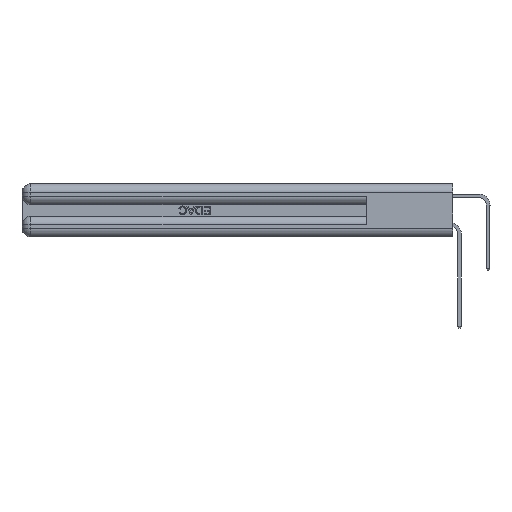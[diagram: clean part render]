
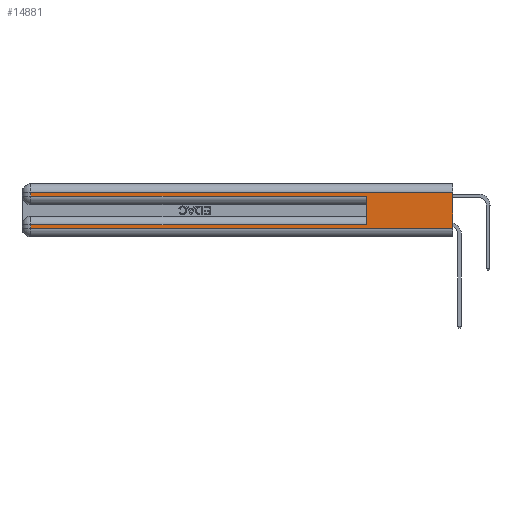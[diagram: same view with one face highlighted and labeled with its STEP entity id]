
A CAD part, left-side view. The second image highlights one B-rep face of the part: STEP entity #14881.
In plain terms, the highlighted planar face has unit normal (-1, 0, 0).
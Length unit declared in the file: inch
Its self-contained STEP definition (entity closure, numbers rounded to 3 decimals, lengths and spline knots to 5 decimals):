
#551 = LINE ( 'NONE', #1925, #33807 ) ;
#1925 = CARTESIAN_POINT ( 'NONE',  ( 0., 0., 0.085 ) ) ;
#4044 = DIRECTION ( 'NONE',  ( 1., 0., 0. ) ) ;
#4581 = CARTESIAN_POINT ( 'NONE',  ( 0., 2.94, 0.31 ) ) ;
#5398 = VERTEX_POINT ( 'NONE', #27032 ) ;
#6913 = LINE ( 'NONE', #38090, #45396 ) ;
#7107 = VERTEX_POINT ( 'NONE', #21104 ) ;
#8309 = CARTESIAN_POINT ( 'NONE',  ( 0., 0., 0.31 ) ) ;
#8334 = ORIENTED_EDGE ( 'NONE', *, *, #34138, .T. ) ;
#8689 = VERTEX_POINT ( 'NONE', #4581 ) ;
#9013 = CARTESIAN_POINT ( 'NONE',  ( 0., 2.94, 0.06 ) ) ;
#9107 = LINE ( 'NONE', #22734, #41726 ) ;
#9156 = VECTOR ( 'NONE', #30788, 39.37008 ) ;
#10543 = EDGE_CURVE ( 'NONE', #7107, #8689, #37160, .T. ) ;
#13018 = DIRECTION ( 'NONE',  ( 0., 1., 0. ) ) ;
#14821 = CARTESIAN_POINT ( 'NONE',  ( 0., 0., 0.37 ) ) ;
#14881 = ADVANCED_FACE ( 'NONE', ( #30387 ), #41164, .F. ) ;
#16146 = DIRECTION ( 'NONE',  ( 0., 0., -1. ) ) ;
#16802 = VERTEX_POINT ( 'NONE', #31632 ) ;
#17012 = VECTOR ( 'NONE', #28247, 39.37008 ) ;
#17228 = ORIENTED_EDGE ( 'NONE', *, *, #10543, .T. ) ;
#17776 = LINE ( 'NONE', #38113, #46366 ) ;
#18522 = VERTEX_POINT ( 'NONE', #23057 ) ;
#19161 = ORIENTED_EDGE ( 'NONE', *, *, #26163, .F. ) ;
#21009 = EDGE_LOOP ( 'NONE', ( #34911, #17228, #40015, #8334, #19161, #46588, #28971, #39958 ) ) ;
#21104 = CARTESIAN_POINT ( 'NONE',  ( 0., 0., 0.31 ) ) ;
#21581 = LINE ( 'NONE', #47509, #40248 ) ;
#22438 = DIRECTION ( 'NONE',  ( 0., 0., -1. ) ) ;
#22734 = CARTESIAN_POINT ( 'NONE',  ( 0., 0., 0.06 ) ) ;
#23057 = CARTESIAN_POINT ( 'NONE',  ( 0., 0.6, 0.085 ) ) ;
#24514 = VERTEX_POINT ( 'NONE', #9013 ) ;
#24845 = AXIS2_PLACEMENT_3D ( 'NONE', #14821, #4044, #22438 ) ;
#25938 = LINE ( 'NONE', #42338, #39953 ) ;
#26163 = EDGE_CURVE ( 'NONE', #18522, #28656, #21581, .T. ) ;
#27032 = CARTESIAN_POINT ( 'NONE',  ( 0., 0., 0.06 ) ) ;
#27153 = EDGE_CURVE ( 'NONE', #7107, #5398, #6913, .T. ) ;
#28247 = DIRECTION ( 'NONE',  ( 0., -1., 0. ) ) ;
#28656 = VERTEX_POINT ( 'NONE', #34473 ) ;
#28904 = DIRECTION ( 'NONE',  ( 0., 0., 1. ) ) ;
#28971 = ORIENTED_EDGE ( 'NONE', *, *, #31458, .T. ) ;
#29905 = DIRECTION ( 'NONE',  ( 0., -1., 0. ) ) ;
#30387 = FACE_OUTER_BOUND ( 'NONE', #21009, .T. ) ;
#30755 = DIRECTION ( 'NONE',  ( 0., 0., -1. ) ) ;
#30788 = DIRECTION ( 'NONE',  ( 0., 1., 0. ) ) ;
#31458 = EDGE_CURVE ( 'NONE', #16802, #24514, #17776, .T. ) ;
#31632 = CARTESIAN_POINT ( 'NONE',  ( 0., 2.94, 0.085 ) ) ;
#33807 = VECTOR ( 'NONE', #13018, 39.37008 ) ;
#34138 = EDGE_CURVE ( 'NONE', #34384, #28656, #35057, .T. ) ;
#34384 = VERTEX_POINT ( 'NONE', #48258 ) ;
#34473 = CARTESIAN_POINT ( 'NONE',  ( 0., 0.6, 0.285 ) ) ;
#34911 = ORIENTED_EDGE ( 'NONE', *, *, #27153, .F. ) ;
#35057 = LINE ( 'NONE', #38888, #17012 ) ;
#37160 = LINE ( 'NONE', #8309, #9156 ) ;
#37734 = EDGE_CURVE ( 'NONE', #18522, #16802, #551, .T. ) ;
#38090 = CARTESIAN_POINT ( 'NONE',  ( 0., 0., 0.37 ) ) ;
#38113 = CARTESIAN_POINT ( 'NONE',  ( 0., 2.94, 0.37 ) ) ;
#38888 = CARTESIAN_POINT ( 'NONE',  ( 0., 0., 0.285 ) ) ;
#39953 = VECTOR ( 'NONE', #46259, 39.37008 ) ;
#39958 = ORIENTED_EDGE ( 'NONE', *, *, #40768, .T. ) ;
#40015 = ORIENTED_EDGE ( 'NONE', *, *, #45877, .T. ) ;
#40248 = VECTOR ( 'NONE', #28904, 39.37008 ) ;
#40768 = EDGE_CURVE ( 'NONE', #24514, #5398, #9107, .T. ) ;
#41164 = PLANE ( 'NONE',  #24845 ) ;
#41726 = VECTOR ( 'NONE', #29905, 39.37008 ) ;
#42338 = CARTESIAN_POINT ( 'NONE',  ( 0., 2.94, 0.37 ) ) ;
#45396 = VECTOR ( 'NONE', #30755, 39.37008 ) ;
#45877 = EDGE_CURVE ( 'NONE', #8689, #34384, #25938, .T. ) ;
#46259 = DIRECTION ( 'NONE',  ( 0., 0., -1. ) ) ;
#46366 = VECTOR ( 'NONE', #16146, 39.37008 ) ;
#46588 = ORIENTED_EDGE ( 'NONE', *, *, #37734, .T. ) ;
#47509 = CARTESIAN_POINT ( 'NONE',  ( 0., 0.6, 0.145 ) ) ;
#48258 = CARTESIAN_POINT ( 'NONE',  ( 0., 2.94, 0.285 ) ) ;
